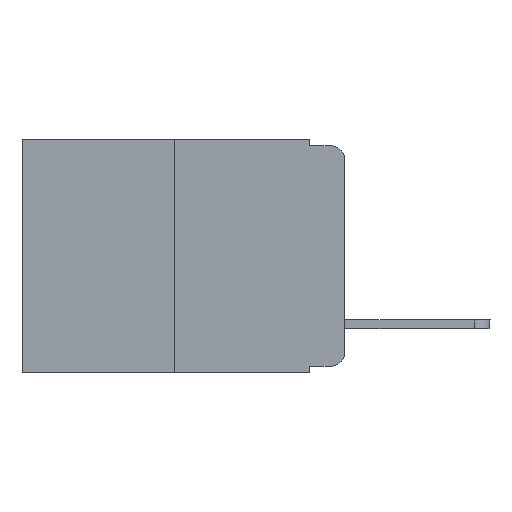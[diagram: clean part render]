
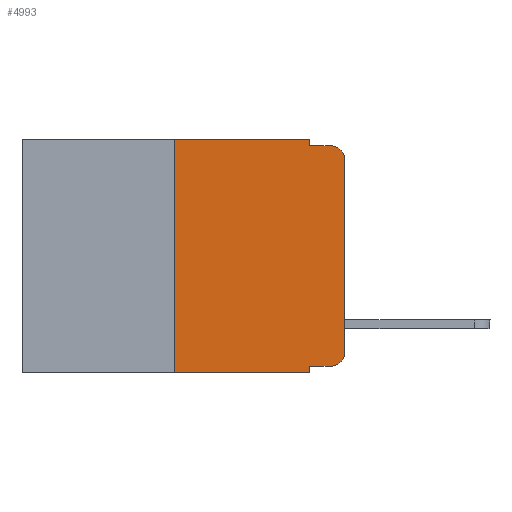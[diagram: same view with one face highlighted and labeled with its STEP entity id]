
A CAD part, left-side view. The second image highlights one B-rep face of the part: STEP entity #4993.
In plain terms, the highlighted planar face has unit normal (-1, 0, 0).
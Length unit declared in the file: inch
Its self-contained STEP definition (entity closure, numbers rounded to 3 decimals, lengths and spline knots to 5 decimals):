
#368 = DIRECTION ( 'NONE',  ( 0., 0., 1. ) ) ;
#375 = VERTEX_POINT ( 'NONE', #3304 ) ;
#700 = DIRECTION ( 'NONE',  ( 0., 0., 1. ) ) ;
#872 = LINE ( 'NONE', #11322, #9806 ) ;
#973 = VERTEX_POINT ( 'NONE', #2761 ) ;
#1188 = ORIENTED_EDGE ( 'NONE', *, *, #15975, .T. ) ;
#1311 = DIRECTION ( 'NONE',  ( 0., 0., -1. ) ) ;
#1527 = CARTESIAN_POINT ( 'NONE',  ( 0., 0.473, 0. ) ) ;
#1536 = VECTOR ( 'NONE', #8097, 39.37008 ) ;
#1818 = EDGE_CURVE ( 'NONE', #7611, #20157, #20047, .T. ) ;
#2325 = CARTESIAN_POINT ( 'NONE',  ( 0., 0.02, -0.313 ) ) ;
#2388 = DIRECTION ( 'NONE',  ( -1., 0., 0. ) ) ;
#2761 = CARTESIAN_POINT ( 'NONE',  ( 0., 0., -0.313 ) ) ;
#2783 = DIRECTION ( 'NONE',  ( 0., -1., 0. ) ) ;
#2798 = LINE ( 'NONE', #15931, #10665 ) ;
#2876 = CARTESIAN_POINT ( 'NONE',  ( 0., 0.051, -0.01 ) ) ;
#3304 = CARTESIAN_POINT ( 'NONE',  ( 0., 0.02, -0.333 ) ) ;
#3404 = CARTESIAN_POINT ( 'NONE',  ( 0., 0., -0.03 ) ) ;
#3458 = CARTESIAN_POINT ( 'NONE',  ( 0., 0.051, -0.343 ) ) ;
#3673 = VECTOR ( 'NONE', #19550, 39.37008 ) ;
#3904 = LINE ( 'NONE', #1527, #1536 ) ;
#4000 = ORIENTED_EDGE ( 'NONE', *, *, #13523, .T. ) ;
#4100 = EDGE_CURVE ( 'NONE', #18611, #375, #14696, .T. ) ;
#4837 = CARTESIAN_POINT ( 'NONE',  ( 0., 0.051, 0. ) ) ;
#4993 = ADVANCED_FACE ( 'NONE', ( #18349 ), #14781, .F. ) ;
#5045 = ORIENTED_EDGE ( 'NONE', *, *, #4100, .T. ) ;
#5724 = CARTESIAN_POINT ( 'NONE',  ( 0., 0.051, 0. ) ) ;
#5762 = VERTEX_POINT ( 'NONE', #3404 ) ;
#5806 = CIRCLE ( 'NONE', #12099, 0.02 ) ;
#6191 = ORIENTED_EDGE ( 'NONE', *, *, #9291, .F. ) ;
#6221 = VECTOR ( 'NONE', #20738, 39.37008 ) ;
#6516 = DIRECTION ( 'NONE',  ( 0., 0., -1. ) ) ;
#6590 = CARTESIAN_POINT ( 'NONE',  ( 0., 0.051, -0.333 ) ) ;
#6906 = CARTESIAN_POINT ( 'NONE',  ( 0., 0.25, 0. ) ) ;
#7611 = VERTEX_POINT ( 'NONE', #17510 ) ;
#7882 = ORIENTED_EDGE ( 'NONE', *, *, #17649, .T. ) ;
#8097 = DIRECTION ( 'NONE',  ( 0., -1., 0. ) ) ;
#9225 = LINE ( 'NONE', #14631, #3673 ) ;
#9291 = EDGE_CURVE ( 'NONE', #14676, #19282, #3904, .T. ) ;
#9671 = LINE ( 'NONE', #17189, #19687 ) ;
#9688 = CARTESIAN_POINT ( 'NONE',  ( 0., 0.473, 0. ) ) ;
#9806 = VECTOR ( 'NONE', #1311, 39.37008 ) ;
#10665 = VECTOR ( 'NONE', #700, 39.37008 ) ;
#11264 = VECTOR ( 'NONE', #11591, 39.37008 ) ;
#11322 = CARTESIAN_POINT ( 'NONE',  ( 0., 0.051, 0. ) ) ;
#11572 = VERTEX_POINT ( 'NONE', #3458 ) ;
#11591 = DIRECTION ( 'NONE',  ( 0., -1., 0. ) ) ;
#11787 = EDGE_LOOP ( 'NONE', ( #7882, #4000, #21697, #17231, #6191, #15315, #13733, #14805, #5045, #1188 ) ) ;
#11971 = EDGE_CURVE ( 'NONE', #19282, #7611, #872, .T. ) ;
#12099 = AXIS2_PLACEMENT_3D ( 'NONE', #2325, #15769, #12540 ) ;
#12540 = DIRECTION ( 'NONE',  ( 0., 0., -1. ) ) ;
#12655 = AXIS2_PLACEMENT_3D ( 'NONE', #9688, #18287, #6516 ) ;
#12910 = CARTESIAN_POINT ( 'NONE',  ( 0., 0.051, -0.333 ) ) ;
#13523 = EDGE_CURVE ( 'NONE', #5762, #20157, #18582, .T. ) ;
#13733 = ORIENTED_EDGE ( 'NONE', *, *, #18040, .T. ) ;
#14009 = EDGE_CURVE ( 'NONE', #20857, #14676, #2798, .T. ) ;
#14072 = DIRECTION ( 'NONE',  ( 0., 0., -1. ) ) ;
#14294 = VECTOR ( 'NONE', #2783, 39.37008 ) ;
#14631 = CARTESIAN_POINT ( 'NONE',  ( 0., 0.473, -0.343 ) ) ;
#14676 = VERTEX_POINT ( 'NONE', #6906 ) ;
#14696 = LINE ( 'NONE', #6590, #11264 ) ;
#14781 = PLANE ( 'NONE',  #12655 ) ;
#14805 = ORIENTED_EDGE ( 'NONE', *, *, #19033, .F. ) ;
#15190 = LINE ( 'NONE', #5724, #6221 ) ;
#15315 = ORIENTED_EDGE ( 'NONE', *, *, #14009, .F. ) ;
#15752 = AXIS2_PLACEMENT_3D ( 'NONE', #20814, #2388, #14072 ) ;
#15769 = DIRECTION ( 'NONE',  ( -1., 0., 0. ) ) ;
#15931 = CARTESIAN_POINT ( 'NONE',  ( 0., 0.25, 0. ) ) ;
#15975 = EDGE_CURVE ( 'NONE', #375, #973, #5806, .T. ) ;
#17189 = CARTESIAN_POINT ( 'NONE',  ( 0., 0., 0. ) ) ;
#17231 = ORIENTED_EDGE ( 'NONE', *, *, #11971, .F. ) ;
#17510 = CARTESIAN_POINT ( 'NONE',  ( 0., 0.051, -0.01 ) ) ;
#17649 = EDGE_CURVE ( 'NONE', #973, #5762, #9671, .T. ) ;
#18040 = EDGE_CURVE ( 'NONE', #20857, #11572, #9225, .T. ) ;
#18287 = DIRECTION ( 'NONE',  ( 1., 0., 0. ) ) ;
#18349 = FACE_OUTER_BOUND ( 'NONE', #11787, .T. ) ;
#18582 = CIRCLE ( 'NONE', #15752, 0.02 ) ;
#18611 = VERTEX_POINT ( 'NONE', #12910 ) ;
#19033 = EDGE_CURVE ( 'NONE', #18611, #11572, #15190, .T. ) ;
#19064 = CARTESIAN_POINT ( 'NONE',  ( 0., 0.02, -0.01 ) ) ;
#19282 = VERTEX_POINT ( 'NONE', #4837 ) ;
#19550 = DIRECTION ( 'NONE',  ( 0., -1., 0. ) ) ;
#19687 = VECTOR ( 'NONE', #368, 39.37008 ) ;
#20047 = LINE ( 'NONE', #2876, #14294 ) ;
#20157 = VERTEX_POINT ( 'NONE', #19064 ) ;
#20701 = CARTESIAN_POINT ( 'NONE',  ( 0., 0.25, -0.343 ) ) ;
#20738 = DIRECTION ( 'NONE',  ( 0., 0., -1. ) ) ;
#20814 = CARTESIAN_POINT ( 'NONE',  ( 0., 0.02, -0.03 ) ) ;
#20857 = VERTEX_POINT ( 'NONE', #20701 ) ;
#21697 = ORIENTED_EDGE ( 'NONE', *, *, #1818, .F. ) ;
